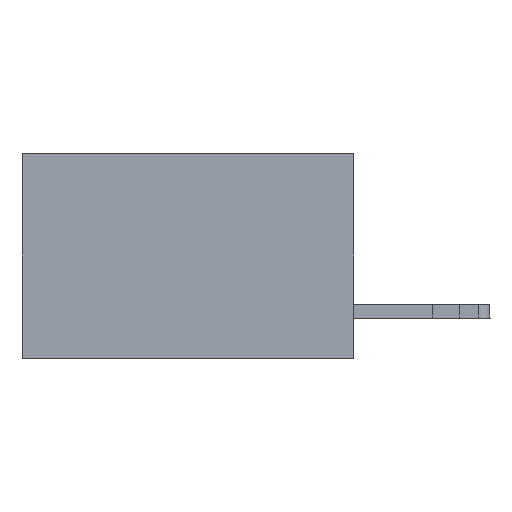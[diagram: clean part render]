
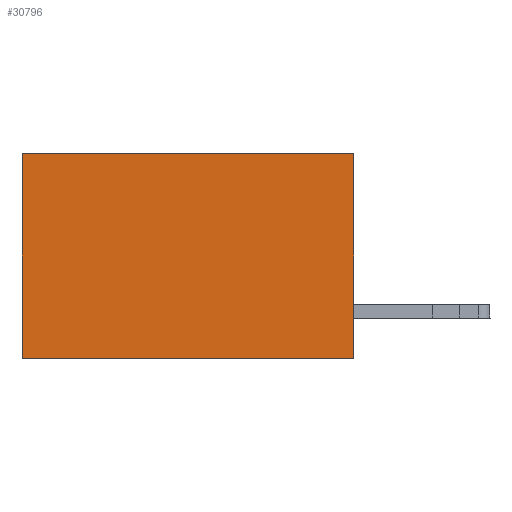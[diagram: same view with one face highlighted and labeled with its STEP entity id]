
A CAD part, left-side view. The second image highlights one B-rep face of the part: STEP entity #30796.
In plain terms, the highlighted planar face has unit normal (-1, 0, 0).
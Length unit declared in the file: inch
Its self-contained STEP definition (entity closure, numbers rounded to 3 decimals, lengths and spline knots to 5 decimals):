
#242 = DIRECTION ( 'NONE',  ( 0., 1., 0. ) ) ;
#1147 = VECTOR ( 'NONE', #18149, 39.37008 ) ;
#1860 = FACE_OUTER_BOUND ( 'NONE', #2027, .T. ) ;
#2027 = EDGE_LOOP ( 'NONE', ( #23734, #7115, #26401, #14078 ) ) ;
#2975 = LINE ( 'NONE', #29099, #33458 ) ;
#3583 = VERTEX_POINT ( 'NONE', #21558 ) ;
#4523 = VERTEX_POINT ( 'NONE', #6287 ) ;
#6247 = CARTESIAN_POINT ( 'NONE',  ( 0.2875, 0., 0. ) ) ;
#6287 = CARTESIAN_POINT ( 'NONE',  ( 0.2875, 0.6, 0. ) ) ;
#6836 = DIRECTION ( 'NONE',  ( 0., 0., -1. ) ) ;
#7115 = ORIENTED_EDGE ( 'NONE', *, *, #16607, .F. ) ;
#7953 = LINE ( 'NONE', #18347, #30518 ) ;
#9152 = LINE ( 'NONE', #29796, #18398 ) ;
#9396 = EDGE_CURVE ( 'NONE', #18640, #30375, #28893, .T. ) ;
#11952 = CARTESIAN_POINT ( 'NONE',  ( 0.2875, 0., 0. ) ) ;
#14078 = ORIENTED_EDGE ( 'NONE', *, *, #26803, .T. ) ;
#16607 = EDGE_CURVE ( 'NONE', #30375, #3583, #7953, .T. ) ;
#18149 = DIRECTION ( 'NONE',  ( 0., 0., -1. ) ) ;
#18347 = CARTESIAN_POINT ( 'NONE',  ( 0.2875, 0., -0.37 ) ) ;
#18398 = VECTOR ( 'NONE', #29301, 39.37008 ) ;
#18640 = VERTEX_POINT ( 'NONE', #6247 ) ;
#19998 = CARTESIAN_POINT ( 'NONE',  ( 0.2875, 0., -0.37 ) ) ;
#20298 = PLANE ( 'NONE',  #30354 ) ;
#21558 = CARTESIAN_POINT ( 'NONE',  ( 0.2875, 0.6, -0.37 ) ) ;
#22346 = DIRECTION ( 'NONE',  ( 1., 0., 0. ) ) ;
#23620 = DIRECTION ( 'NONE',  ( 0., 1., 0. ) ) ;
#23734 = ORIENTED_EDGE ( 'NONE', *, *, #32847, .T. ) ;
#26401 = ORIENTED_EDGE ( 'NONE', *, *, #9396, .F. ) ;
#26803 = EDGE_CURVE ( 'NONE', #18640, #4523, #2975, .T. ) ;
#28728 = CARTESIAN_POINT ( 'NONE',  ( 0.2875, 0., 0. ) ) ;
#28893 = LINE ( 'NONE', #28728, #1147 ) ;
#29099 = CARTESIAN_POINT ( 'NONE',  ( 0.2875, 0., 0. ) ) ;
#29301 = DIRECTION ( 'NONE',  ( 0., 0., -1. ) ) ;
#29796 = CARTESIAN_POINT ( 'NONE',  ( 0.2875, 0.6, 0. ) ) ;
#30354 = AXIS2_PLACEMENT_3D ( 'NONE', #11952, #22346, #6836 ) ;
#30375 = VERTEX_POINT ( 'NONE', #19998 ) ;
#30518 = VECTOR ( 'NONE', #242, 39.37008 ) ;
#30796 = ADVANCED_FACE ( 'NONE', ( #1860 ), #20298, .F. ) ;
#32847 = EDGE_CURVE ( 'NONE', #4523, #3583, #9152, .T. ) ;
#33458 = VECTOR ( 'NONE', #23620, 39.37008 ) ;
